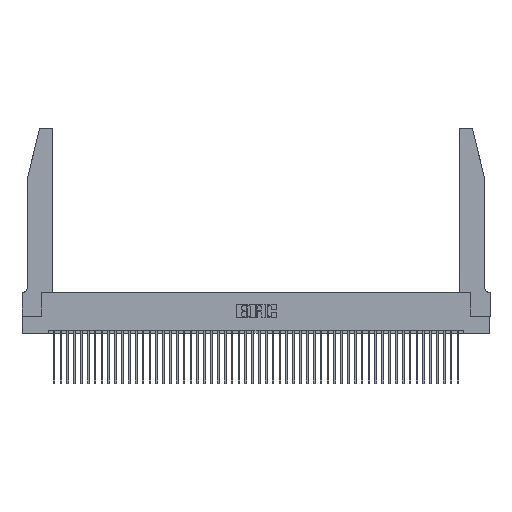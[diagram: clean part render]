
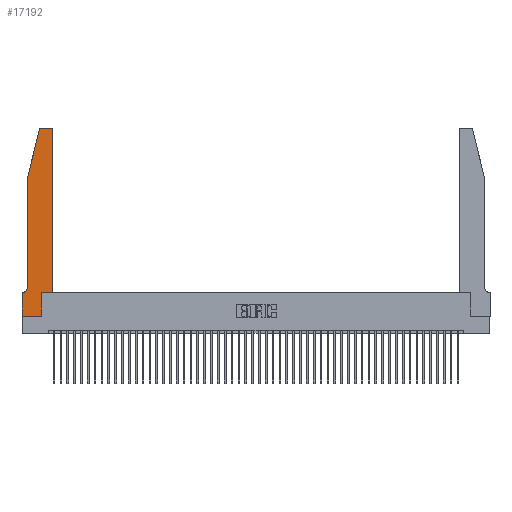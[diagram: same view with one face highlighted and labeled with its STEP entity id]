
A CAD part, top view. The second image highlights one B-rep face of the part: STEP entity #17192.
In plain terms, the highlighted planar face has unit normal (0, 0, 1).
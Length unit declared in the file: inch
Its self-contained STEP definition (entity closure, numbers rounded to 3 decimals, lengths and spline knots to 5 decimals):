
#709 = CARTESIAN_POINT ( 'NONE',  ( 0.0055, 0.35, 0.37 ) ) ;
#1334 = VERTEX_POINT ( 'NONE', #17856 ) ;
#1454 = DIRECTION ( 'NONE',  ( 0., 0., 1. ) ) ;
#1949 = VECTOR ( 'NONE', #31287, 39.37008 ) ;
#2000 = LINE ( 'NONE', #42857, #31473 ) ;
#2112 = CARTESIAN_POINT ( 'NONE',  ( 0.0755, 0.42, 0.37 ) ) ;
#2905 = LINE ( 'NONE', #25197, #42427 ) ;
#3400 = CARTESIAN_POINT ( 'NONE',  ( 0.284, 2.75, 0.37 ) ) ;
#3565 = DIRECTION ( 'NONE',  ( 0., 0., 1. ) ) ;
#5052 = CARTESIAN_POINT ( 'NONE',  ( 0.4505, 0.35, 0.37 ) ) ;
#5247 = ORIENTED_EDGE ( 'NONE', *, *, #37856, .T. ) ;
#6279 = CARTESIAN_POINT ( 'NONE',  ( 0., 0., 0.37 ) ) ;
#6341 = DIRECTION ( 'NONE',  ( 0., -1., 0. ) ) ;
#6356 = VECTOR ( 'NONE', #6341, 39.37008 ) ;
#6423 = EDGE_CURVE ( 'NONE', #47663, #17350, #17874, .T. ) ;
#6838 = DIRECTION ( 'NONE',  ( -1., 0., 0. ) ) ;
#6998 = EDGE_CURVE ( 'NONE', #31623, #1334, #33297, .T. ) ;
#8798 = VECTOR ( 'NONE', #24760, 39.37008 ) ;
#8856 = ORIENTED_EDGE ( 'NONE', *, *, #35631, .T. ) ;
#9853 = CARTESIAN_POINT ( 'NONE',  ( 0.2865, 0.35, 0.37 ) ) ;
#10298 = CARTESIAN_POINT ( 'NONE',  ( 0.2865, 0.35, 0.37 ) ) ;
#10695 = ORIENTED_EDGE ( 'NONE', *, *, #48126, .T. ) ;
#11778 = EDGE_CURVE ( 'NONE', #17350, #31623, #32366, .T. ) ;
#12378 = CARTESIAN_POINT ( 'NONE',  ( 0.4205, 2.75, 0.37 ) ) ;
#13437 = CARTESIAN_POINT ( 'NONE',  ( 0.0755, 0.35, 0.37 ) ) ;
#13764 = DIRECTION ( 'NONE',  ( -1., 0., 0. ) ) ;
#15891 = CARTESIAN_POINT ( 'NONE',  ( 0.2865, 0., 0.37 ) ) ;
#16508 = VERTEX_POINT ( 'NONE', #5052 ) ;
#16791 = CARTESIAN_POINT ( 'NONE',  ( 0.0055, 0.42, 0.37 ) ) ;
#16867 = CARTESIAN_POINT ( 'NONE',  ( 0.4205, 2.72, 0.37 ) ) ;
#17192 = ADVANCED_FACE ( 'NONE', ( #36005 ), #20682, .T. ) ;
#17350 = VERTEX_POINT ( 'NONE', #2112 ) ;
#17856 = CARTESIAN_POINT ( 'NONE',  ( 0., 0.35, 0.37 ) ) ;
#17874 = LINE ( 'NONE', #21679, #6356 ) ;
#19489 = CIRCLE ( 'NONE', #39864, 0.03 ) ;
#19946 = ORIENTED_EDGE ( 'NONE', *, *, #46154, .T. ) ;
#19947 = ORIENTED_EDGE ( 'NONE', *, *, #26192, .T. ) ;
#20143 = ORIENTED_EDGE ( 'NONE', *, *, #39412, .T. ) ;
#20575 = DIRECTION ( 'NONE',  ( -1., 0., 0. ) ) ;
#20661 = DIRECTION ( 'NONE',  ( 1., 0., 0. ) ) ;
#20682 = PLANE ( 'NONE',  #29750 ) ;
#20746 = DIRECTION ( 'NONE',  ( 1., 0., 0. ) ) ;
#21679 = CARTESIAN_POINT ( 'NONE',  ( 0.0755, 2., 0.37 ) ) ;
#23675 = LINE ( 'NONE', #27465, #1949 ) ;
#24662 = VERTEX_POINT ( 'NONE', #29394 ) ;
#24760 = DIRECTION ( 'NONE',  ( 0., 1., 0. ) ) ;
#25197 = CARTESIAN_POINT ( 'NONE',  ( 0.4505, 0.35, 0.37 ) ) ;
#25849 = CARTESIAN_POINT ( 'NONE',  ( 0.2605, 2.75, 0.37 ) ) ;
#26192 = EDGE_CURVE ( 'NONE', #47055, #45680, #28793, .T. ) ;
#26636 = CARTESIAN_POINT ( 'NONE',  ( 0.284, 2.72, 0.37 ) ) ;
#26739 = VERTEX_POINT ( 'NONE', #12378 ) ;
#27465 = CARTESIAN_POINT ( 'NONE',  ( 0., 0., 0.37 ) ) ;
#27965 = DIRECTION ( 'NONE',  ( -0.239, -0.971, 0. ) ) ;
#28382 = DIRECTION ( 'NONE',  ( 1., 0., 0. ) ) ;
#28793 = LINE ( 'NONE', #43519, #48861 ) ;
#29222 = LINE ( 'NONE', #47417, #8798 ) ;
#29394 = CARTESIAN_POINT ( 'NONE',  ( 0.25487, 2.72718, 0.37 ) ) ;
#29750 = AXIS2_PLACEMENT_3D ( 'NONE', #47204, #1454, #28382 ) ;
#29757 = VECTOR ( 'NONE', #32762, 39.37008 ) ;
#29803 = VERTEX_POINT ( 'NONE', #3400 ) ;
#29984 = EDGE_CURVE ( 'NONE', #24662, #47663, #2000, .T. ) ;
#30072 = CIRCLE ( 'NONE', #34719, 0.03 ) ;
#30455 = DIRECTION ( 'NONE',  ( 1., 0., 0. ) ) ;
#31287 = DIRECTION ( 'NONE',  ( 0., -1., 0. ) ) ;
#31473 = VECTOR ( 'NONE', #27965, 39.37008 ) ;
#31623 = VERTEX_POINT ( 'NONE', #709 ) ;
#32166 = AXIS2_PLACEMENT_3D ( 'NONE', #16791, #43340, #20575 ) ;
#32366 = CIRCLE ( 'NONE', #32166, 0.07 ) ;
#32762 = DIRECTION ( 'NONE',  ( 0., 1., 0. ) ) ;
#33297 = LINE ( 'NONE', #13437, #42164 ) ;
#33871 = VECTOR ( 'NONE', #6838, 39.37008 ) ;
#34494 = VERTEX_POINT ( 'NONE', #10298 ) ;
#34719 = AXIS2_PLACEMENT_3D ( 'NONE', #16867, #43427, #20661 ) ;
#35631 = EDGE_CURVE ( 'NONE', #45680, #34494, #39830, .T. ) ;
#35758 = ORIENTED_EDGE ( 'NONE', *, *, #11778, .T. ) ;
#35767 = ORIENTED_EDGE ( 'NONE', *, *, #6998, .T. ) ;
#35786 = EDGE_LOOP ( 'NONE', ( #19946, #20143, #45827, #48305, #35758, #35767, #39426, #19947, #8856, #48080, #5247, #10695 ) ) ;
#36005 = FACE_OUTER_BOUND ( 'NONE', #35786, .T. ) ;
#37856 = EDGE_CURVE ( 'NONE', #16508, #48967, #29222, .T. ) ;
#39412 = EDGE_CURVE ( 'NONE', #29803, #24662, #19489, .T. ) ;
#39426 = ORIENTED_EDGE ( 'NONE', *, *, #39598, .T. ) ;
#39598 = EDGE_CURVE ( 'NONE', #1334, #47055, #23675, .T. ) ;
#39830 = LINE ( 'NONE', #9853, #29757 ) ;
#39864 = AXIS2_PLACEMENT_3D ( 'NONE', #26636, #3565, #30455 ) ;
#40813 = CARTESIAN_POINT ( 'NONE',  ( 0.0755, 2., 0.37 ) ) ;
#41858 = EDGE_CURVE ( 'NONE', #34494, #16508, #2905, .T. ) ;
#42164 = VECTOR ( 'NONE', #13764, 39.37008 ) ;
#42427 = VECTOR ( 'NONE', #47846, 39.37008 ) ;
#42857 = CARTESIAN_POINT ( 'NONE',  ( 0.0755, 2., 0.37 ) ) ;
#43340 = DIRECTION ( 'NONE',  ( 0., 0., -1. ) ) ;
#43427 = DIRECTION ( 'NONE',  ( 0., 0., 1. ) ) ;
#43519 = CARTESIAN_POINT ( 'NONE',  ( 0., 0., 0.37 ) ) ;
#43925 = LINE ( 'NONE', #25849, #33871 ) ;
#45680 = VERTEX_POINT ( 'NONE', #15891 ) ;
#45827 = ORIENTED_EDGE ( 'NONE', *, *, #29984, .T. ) ;
#46154 = EDGE_CURVE ( 'NONE', #26739, #29803, #43925, .T. ) ;
#47055 = VERTEX_POINT ( 'NONE', #6279 ) ;
#47204 = CARTESIAN_POINT ( 'NONE',  ( 0., 0.35, 0.37 ) ) ;
#47417 = CARTESIAN_POINT ( 'NONE',  ( 0.4505, 0.35, 0.37 ) ) ;
#47446 = CARTESIAN_POINT ( 'NONE',  ( 0.4505, 2.72, 0.37 ) ) ;
#47663 = VERTEX_POINT ( 'NONE', #40813 ) ;
#47846 = DIRECTION ( 'NONE',  ( 1., 0., 0. ) ) ;
#48080 = ORIENTED_EDGE ( 'NONE', *, *, #41858, .T. ) ;
#48126 = EDGE_CURVE ( 'NONE', #48967, #26739, #30072, .T. ) ;
#48305 = ORIENTED_EDGE ( 'NONE', *, *, #6423, .T. ) ;
#48861 = VECTOR ( 'NONE', #20746, 39.37008 ) ;
#48967 = VERTEX_POINT ( 'NONE', #47446 ) ;
